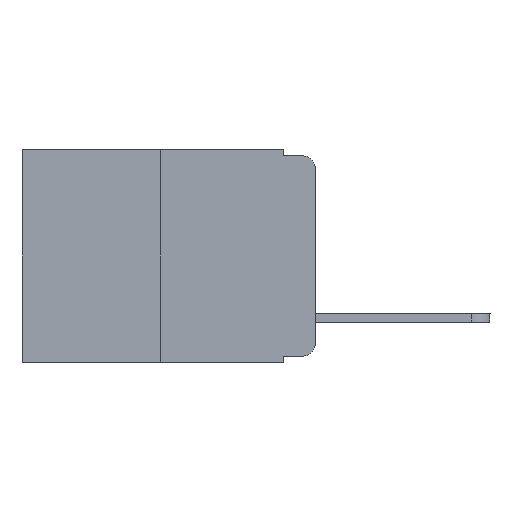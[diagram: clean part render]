
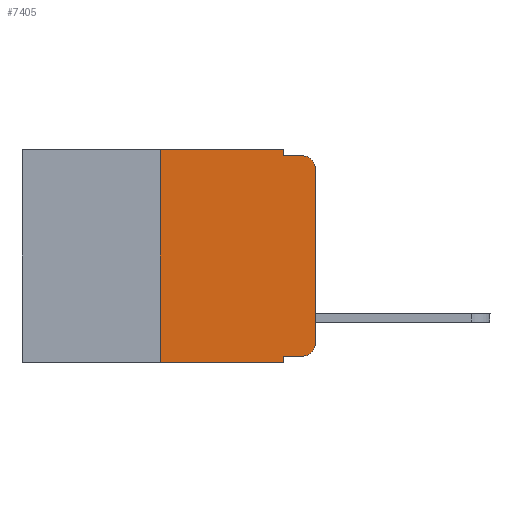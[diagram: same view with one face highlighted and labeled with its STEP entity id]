
A CAD part, left-side view. The second image highlights one B-rep face of the part: STEP entity #7405.
In plain terms, the highlighted planar face has unit normal (-1, 0, 0).
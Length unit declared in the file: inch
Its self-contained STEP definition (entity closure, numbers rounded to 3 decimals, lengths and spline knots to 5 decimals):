
#56 = VERTEX_POINT ( 'NONE', #9240 ) ;
#148 = ORIENTED_EDGE ( 'NONE', *, *, #9815, .T. ) ;
#187 = VERTEX_POINT ( 'NONE', #4771 ) ;
#467 = EDGE_CURVE ( 'NONE', #10263, #9978, #4694, .T. ) ;
#675 = ORIENTED_EDGE ( 'NONE', *, *, #1772, .T. ) ;
#696 = VERTEX_POINT ( 'NONE', #6796 ) ;
#1117 = CARTESIAN_POINT ( 'NONE',  ( 0., 0.473, 0. ) ) ;
#1407 = ORIENTED_EDGE ( 'NONE', *, *, #9561, .F. ) ;
#1726 = EDGE_CURVE ( 'NONE', #2751, #10780, #10683, .T. ) ;
#1727 = CARTESIAN_POINT ( 'NONE',  ( 0., 0.473, 0. ) ) ;
#1772 = EDGE_CURVE ( 'NONE', #2751, #3187, #9095, .T. ) ;
#1963 = ORIENTED_EDGE ( 'NONE', *, *, #1726, .F. ) ;
#2017 = CARTESIAN_POINT ( 'NONE',  ( 0., 0.051, -0.333 ) ) ;
#2077 = CARTESIAN_POINT ( 'NONE',  ( 0., 0.25, -0.343 ) ) ;
#2373 = CARTESIAN_POINT ( 'NONE',  ( 0., 0.473, -0.343 ) ) ;
#2469 = ORIENTED_EDGE ( 'NONE', *, *, #5043, .F. ) ;
#2751 = VERTEX_POINT ( 'NONE', #2077 ) ;
#2958 = VERTEX_POINT ( 'NONE', #8182 ) ;
#2961 = VECTOR ( 'NONE', #5773, 39.37008 ) ;
#3131 = CARTESIAN_POINT ( 'NONE',  ( 0., 0.25, 0. ) ) ;
#3187 = VERTEX_POINT ( 'NONE', #10566 ) ;
#3218 = CARTESIAN_POINT ( 'NONE',  ( 0., 0.02, -0.333 ) ) ;
#3341 = CARTESIAN_POINT ( 'NONE',  ( 0., 0.051, 0. ) ) ;
#3751 = DIRECTION ( 'NONE',  ( 0., 0., 1. ) ) ;
#3827 = ORIENTED_EDGE ( 'NONE', *, *, #10614, .F. ) ;
#3846 = LINE ( 'NONE', #10717, #6365 ) ;
#3855 = EDGE_CURVE ( 'NONE', #56, #696, #9459, .T. ) ;
#4113 = EDGE_CURVE ( 'NONE', #10780, #5997, #8770, .T. ) ;
#4217 = CARTESIAN_POINT ( 'NONE',  ( 0., 0.051, -0.01 ) ) ;
#4247 = VECTOR ( 'NONE', #8616, 39.37008 ) ;
#4509 = CARTESIAN_POINT ( 'NONE',  ( 0., 0., 0. ) ) ;
#4694 = LINE ( 'NONE', #2017, #7524 ) ;
#4723 = DIRECTION ( 'NONE',  ( 0., 0., -1. ) ) ;
#4771 = CARTESIAN_POINT ( 'NONE',  ( 0., 0.02, -0.01 ) ) ;
#5043 = EDGE_CURVE ( 'NONE', #2958, #187, #10226, .T. ) ;
#5107 = PLANE ( 'NONE',  #6130 ) ;
#5161 = DIRECTION ( 'NONE',  ( 1., 0., 0. ) ) ;
#5377 = ORIENTED_EDGE ( 'NONE', *, *, #6341, .T. ) ;
#5420 = VECTOR ( 'NONE', #3751, 39.37008 ) ;
#5552 = DIRECTION ( 'NONE',  ( -1., 0., 0. ) ) ;
#5773 = DIRECTION ( 'NONE',  ( 0., -1., 0. ) ) ;
#5885 = EDGE_LOOP ( 'NONE', ( #9175, #148, #2469, #3827, #5952, #1963, #675, #1407, #7521, #5377 ) ) ;
#5952 = ORIENTED_EDGE ( 'NONE', *, *, #4113, .F. ) ;
#5997 = VERTEX_POINT ( 'NONE', #6979 ) ;
#6130 = AXIS2_PLACEMENT_3D ( 'NONE', #1727, #5161, #9423 ) ;
#6177 = AXIS2_PLACEMENT_3D ( 'NONE', #7403, #6350, #4723 ) ;
#6341 = EDGE_CURVE ( 'NONE', #9978, #56, #9126, .T. ) ;
#6350 = DIRECTION ( 'NONE',  ( -1., 0., 0. ) ) ;
#6365 = VECTOR ( 'NONE', #7831, 39.37008 ) ;
#6439 = CARTESIAN_POINT ( 'NONE',  ( 0., 0.25, 0. ) ) ;
#6696 = VECTOR ( 'NONE', #6733, 39.37008 ) ;
#6733 = DIRECTION ( 'NONE',  ( 0., 0., -1. ) ) ;
#6796 = CARTESIAN_POINT ( 'NONE',  ( 0., 0., -0.03 ) ) ;
#6979 = CARTESIAN_POINT ( 'NONE',  ( 0., 0.051, 0. ) ) ;
#7403 = CARTESIAN_POINT ( 'NONE',  ( 0., 0.02, -0.03 ) ) ;
#7405 = ADVANCED_FACE ( 'NONE', ( #9376 ), #5107, .F. ) ;
#7521 = ORIENTED_EDGE ( 'NONE', *, *, #467, .T. ) ;
#7524 = VECTOR ( 'NONE', #10608, 39.37008 ) ;
#7831 = DIRECTION ( 'NONE',  ( 0., 0., -1. ) ) ;
#7839 = DIRECTION ( 'NONE',  ( 0., -1., 0. ) ) ;
#7986 = VECTOR ( 'NONE', #7839, 39.37008 ) ;
#8182 = CARTESIAN_POINT ( 'NONE',  ( 0., 0.051, -0.01 ) ) ;
#8616 = DIRECTION ( 'NONE',  ( 0., 0., 1. ) ) ;
#8770 = LINE ( 'NONE', #1117, #7986 ) ;
#8819 = CARTESIAN_POINT ( 'NONE',  ( 0., 0.051, -0.333 ) ) ;
#8926 = AXIS2_PLACEMENT_3D ( 'NONE', #9774, #5552, #10690 ) ;
#9095 = LINE ( 'NONE', #2373, #9148 ) ;
#9126 = CIRCLE ( 'NONE', #8926, 0.02 ) ;
#9148 = VECTOR ( 'NONE', #9941, 39.37008 ) ;
#9175 = ORIENTED_EDGE ( 'NONE', *, *, #3855, .T. ) ;
#9240 = CARTESIAN_POINT ( 'NONE',  ( 0., 0., -0.313 ) ) ;
#9376 = FACE_OUTER_BOUND ( 'NONE', #5885, .T. ) ;
#9423 = DIRECTION ( 'NONE',  ( 0., 0., -1. ) ) ;
#9459 = LINE ( 'NONE', #4509, #4247 ) ;
#9561 = EDGE_CURVE ( 'NONE', #10263, #3187, #10022, .T. ) ;
#9774 = CARTESIAN_POINT ( 'NONE',  ( 0., 0.02, -0.313 ) ) ;
#9815 = EDGE_CURVE ( 'NONE', #696, #187, #10449, .T. ) ;
#9941 = DIRECTION ( 'NONE',  ( 0., -1., 0. ) ) ;
#9978 = VERTEX_POINT ( 'NONE', #3218 ) ;
#10022 = LINE ( 'NONE', #3341, #6696 ) ;
#10226 = LINE ( 'NONE', #4217, #2961 ) ;
#10263 = VERTEX_POINT ( 'NONE', #8819 ) ;
#10449 = CIRCLE ( 'NONE', #6177, 0.02 ) ;
#10566 = CARTESIAN_POINT ( 'NONE',  ( 0., 0.051, -0.343 ) ) ;
#10608 = DIRECTION ( 'NONE',  ( 0., -1., 0. ) ) ;
#10614 = EDGE_CURVE ( 'NONE', #5997, #2958, #3846, .T. ) ;
#10683 = LINE ( 'NONE', #6439, #5420 ) ;
#10690 = DIRECTION ( 'NONE',  ( 0., 0., -1. ) ) ;
#10717 = CARTESIAN_POINT ( 'NONE',  ( 0., 0.051, 0. ) ) ;
#10780 = VERTEX_POINT ( 'NONE', #3131 ) ;
